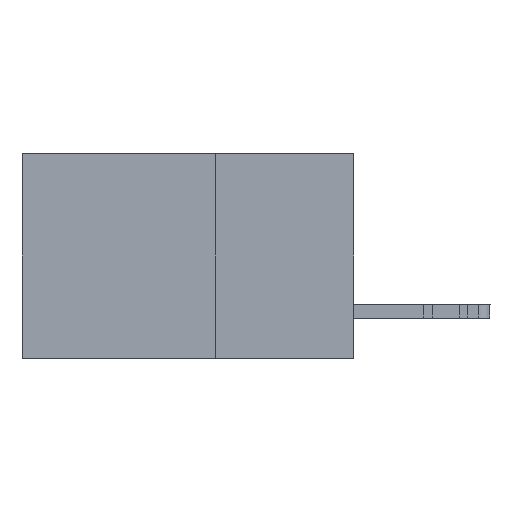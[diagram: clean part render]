
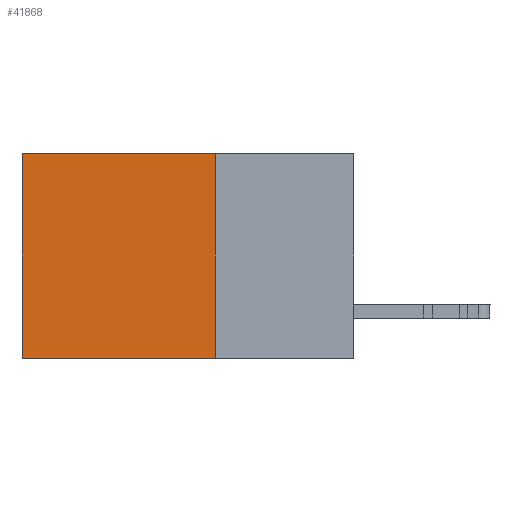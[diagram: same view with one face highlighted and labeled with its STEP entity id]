
A CAD part, left-side view. The second image highlights one B-rep face of the part: STEP entity #41868.
In plain terms, the highlighted planar face has unit normal (-1, 0, 0).
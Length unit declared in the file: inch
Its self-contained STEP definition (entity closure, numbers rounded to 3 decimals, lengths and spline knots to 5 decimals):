
#3407 = VERTEX_POINT ( 'NONE', #4874 ) ;
#4752 = ORIENTED_EDGE ( 'NONE', *, *, #10670, .F. ) ;
#4874 = CARTESIAN_POINT ( 'NONE',  ( 0.2875, 0.25, 0. ) ) ;
#5217 = CARTESIAN_POINT ( 'NONE',  ( 0.2875, 0.25, -0.37 ) ) ;
#6144 = EDGE_CURVE ( 'NONE', #3407, #11686, #22447, .T. ) ;
#7114 = VECTOR ( 'NONE', #30268, 39.37008 ) ;
#8053 = VERTEX_POINT ( 'NONE', #37318 ) ;
#10670 = EDGE_CURVE ( 'NONE', #3407, #31096, #24444, .T. ) ;
#11468 = DIRECTION ( 'NONE',  ( 0., 0., -1. ) ) ;
#11686 = VERTEX_POINT ( 'NONE', #41653 ) ;
#12496 = EDGE_CURVE ( 'NONE', #31096, #8053, #37683, .T. ) ;
#12696 = CARTESIAN_POINT ( 'NONE',  ( 0.2875, 0.25, 0. ) ) ;
#14522 = ORIENTED_EDGE ( 'NONE', *, *, #6144, .T. ) ;
#14787 = CARTESIAN_POINT ( 'NONE',  ( 0.2875, 0.25, 0. ) ) ;
#15311 = PLANE ( 'NONE',  #33963 ) ;
#16804 = VECTOR ( 'NONE', #39514, 39.37008 ) ;
#22447 = LINE ( 'NONE', #14787, #44964 ) ;
#22928 = DIRECTION ( 'NONE',  ( 0., 1., 0. ) ) ;
#24444 = LINE ( 'NONE', #12696, #32565 ) ;
#24604 = LINE ( 'NONE', #39263, #16804 ) ;
#25490 = EDGE_LOOP ( 'NONE', ( #30764, #40604, #4752, #14522 ) ) ;
#26681 = EDGE_CURVE ( 'NONE', #11686, #8053, #24604, .T. ) ;
#27349 = DIRECTION ( 'NONE',  ( 0., 0., -1. ) ) ;
#29257 = FACE_OUTER_BOUND ( 'NONE', #25490, .T. ) ;
#30268 = DIRECTION ( 'NONE',  ( 0., 1., 0. ) ) ;
#30764 = ORIENTED_EDGE ( 'NONE', *, *, #26681, .T. ) ;
#30934 = CARTESIAN_POINT ( 'NONE',  ( 0.2875, 0.25, -0.37 ) ) ;
#31096 = VERTEX_POINT ( 'NONE', #30934 ) ;
#32565 = VECTOR ( 'NONE', #27349, 39.37008 ) ;
#32887 = CARTESIAN_POINT ( 'NONE',  ( 0.2875, 0.25, 0. ) ) ;
#33356 = DIRECTION ( 'NONE',  ( 1., 0., 0. ) ) ;
#33963 = AXIS2_PLACEMENT_3D ( 'NONE', #32887, #33356, #11468 ) ;
#37318 = CARTESIAN_POINT ( 'NONE',  ( 0.2875, 0.6, -0.37 ) ) ;
#37683 = LINE ( 'NONE', #5217, #7114 ) ;
#39263 = CARTESIAN_POINT ( 'NONE',  ( 0.2875, 0.6, 0. ) ) ;
#39514 = DIRECTION ( 'NONE',  ( 0., 0., -1. ) ) ;
#40604 = ORIENTED_EDGE ( 'NONE', *, *, #12496, .F. ) ;
#41653 = CARTESIAN_POINT ( 'NONE',  ( 0.2875, 0.6, 0. ) ) ;
#41868 = ADVANCED_FACE ( 'NONE', ( #29257 ), #15311, .F. ) ;
#44964 = VECTOR ( 'NONE', #22928, 39.37008 ) ;
